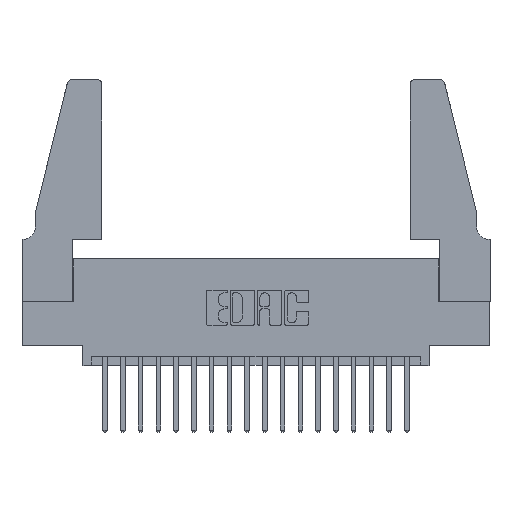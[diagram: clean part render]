
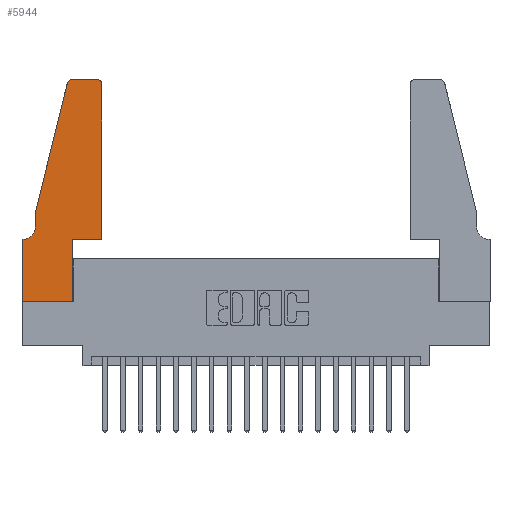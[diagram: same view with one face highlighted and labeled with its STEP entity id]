
A CAD part, top view. The second image highlights one B-rep face of the part: STEP entity #5944.
In plain terms, the highlighted planar face has unit normal (0, 0, 1).
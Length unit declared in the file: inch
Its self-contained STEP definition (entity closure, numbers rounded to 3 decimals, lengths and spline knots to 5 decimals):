
#73 = CARTESIAN_POINT ( 'NONE',  ( 0.2605, 1.25, 0.37 ) ) ;
#491 = DIRECTION ( 'NONE',  ( 0., -1., 0. ) ) ;
#494 = LINE ( 'NONE', #3591, #12289 ) ;
#753 = CARTESIAN_POINT ( 'NONE',  ( 0.2865, 0.35, 0.37 ) ) ;
#868 = CARTESIAN_POINT ( 'NONE',  ( 0.284, 1.22, 0.37 ) ) ;
#1117 = DIRECTION ( 'NONE',  ( -1., 0., 0. ) ) ;
#1159 = LINE ( 'NONE', #73, #8864 ) ;
#1580 = LINE ( 'NONE', #13448, #9281 ) ;
#1698 = DIRECTION ( 'NONE',  ( 0., 1., 0. ) ) ;
#1801 = ORIENTED_EDGE ( 'NONE', *, *, #15707, .T. ) ;
#1884 = CARTESIAN_POINT ( 'NONE',  ( 0.2865, 0., 0.37 ) ) ;
#2112 = ORIENTED_EDGE ( 'NONE', *, *, #2718, .T. ) ;
#2433 = DIRECTION ( 'NONE',  ( 1., 0., 0. ) ) ;
#2710 = DIRECTION ( 'NONE',  ( 0., 1., 0. ) ) ;
#2718 = EDGE_CURVE ( 'NONE', #13651, #10757, #12244, .T. ) ;
#3139 = DIRECTION ( 'NONE',  ( -1., 0., 0. ) ) ;
#3528 = ORIENTED_EDGE ( 'NONE', *, *, #18840, .T. ) ;
#3591 = CARTESIAN_POINT ( 'NONE',  ( 0., 0., 0.37 ) ) ;
#3637 = AXIS2_PLACEMENT_3D ( 'NONE', #19285, #10341, #1117 ) ;
#3677 = CARTESIAN_POINT ( 'NONE',  ( 0.4205, 1.22, 0.37 ) ) ;
#3993 = CARTESIAN_POINT ( 'NONE',  ( 0.0755, 0.5, 0.37 ) ) ;
#4650 = ORIENTED_EDGE ( 'NONE', *, *, #13378, .T. ) ;
#4763 = CARTESIAN_POINT ( 'NONE',  ( 0.4505, 0.35, 0.37 ) ) ;
#4810 = EDGE_CURVE ( 'NONE', #14926, #13351, #1580, .T. ) ;
#5226 = DIRECTION ( 'NONE',  ( 1., 0., 0. ) ) ;
#5566 = DIRECTION ( 'NONE',  ( 0., -1., 0. ) ) ;
#5788 = DIRECTION ( 'NONE',  ( -0.239, -0.971, 0. ) ) ;
#5944 = ADVANCED_FACE ( 'NONE', ( #18175 ), #12454, .T. ) ;
#6122 = VECTOR ( 'NONE', #19606, 39.37008 ) ;
#6267 = AXIS2_PLACEMENT_3D ( 'NONE', #3677, #14351, #5226 ) ;
#6272 = CARTESIAN_POINT ( 'NONE',  ( 0.2865, 0.35, 0.37 ) ) ;
#6332 = DIRECTION ( 'NONE',  ( 1., 0., 0. ) ) ;
#6452 = CARTESIAN_POINT ( 'NONE',  ( 0., 0.35, 0.37 ) ) ;
#6780 = ORIENTED_EDGE ( 'NONE', *, *, #13356, .T. ) ;
#7181 = CARTESIAN_POINT ( 'NONE',  ( 0.4205, 1.25, 0.37 ) ) ;
#7207 = AXIS2_PLACEMENT_3D ( 'NONE', #13944, #15433, #6332 ) ;
#7335 = EDGE_CURVE ( 'NONE', #10085, #14926, #16744, .T. ) ;
#7605 = LINE ( 'NONE', #14009, #10738 ) ;
#8207 = VERTEX_POINT ( 'NONE', #18926 ) ;
#8531 = CARTESIAN_POINT ( 'NONE',  ( 0.0755, 0.42, 0.37 ) ) ;
#8585 = VERTEX_POINT ( 'NONE', #10897 ) ;
#8630 = VECTOR ( 'NONE', #5566, 39.37008 ) ;
#8864 = VECTOR ( 'NONE', #3139, 39.37008 ) ;
#8877 = CARTESIAN_POINT ( 'NONE',  ( 0.4505, 0.35, 0.37 ) ) ;
#9092 = ORIENTED_EDGE ( 'NONE', *, *, #14927, .T. ) ;
#9281 = VECTOR ( 'NONE', #2710, 39.37008 ) ;
#9376 = DIRECTION ( 'NONE',  ( 1., 0., 0. ) ) ;
#9969 = EDGE_CURVE ( 'NONE', #12098, #10286, #494, .T. ) ;
#10085 = VERTEX_POINT ( 'NONE', #753 ) ;
#10138 = ORIENTED_EDGE ( 'NONE', *, *, #7335, .T. ) ;
#10286 = VERTEX_POINT ( 'NONE', #19382 ) ;
#10341 = DIRECTION ( 'NONE',  ( 0., 0., -1. ) ) ;
#10649 = VECTOR ( 'NONE', #9376, 39.37008 ) ;
#10738 = VECTOR ( 'NONE', #15509, 39.37008 ) ;
#10757 = VERTEX_POINT ( 'NONE', #8531 ) ;
#10801 = ORIENTED_EDGE ( 'NONE', *, *, #17772, .T. ) ;
#10897 = CARTESIAN_POINT ( 'NONE',  ( 0.25487, 1.22718, 0.37 ) ) ;
#11215 = VECTOR ( 'NONE', #1698, 39.37008 ) ;
#11423 = ORIENTED_EDGE ( 'NONE', *, *, #4810, .T. ) ;
#11634 = DIRECTION ( 'NONE',  ( 0., 0., 1. ) ) ;
#11692 = LINE ( 'NONE', #6272, #11215 ) ;
#11838 = ORIENTED_EDGE ( 'NONE', *, *, #9969, .T. ) ;
#12098 = VERTEX_POINT ( 'NONE', #6452 ) ;
#12122 = CIRCLE ( 'NONE', #15082, 0.03 ) ;
#12153 = ORIENTED_EDGE ( 'NONE', *, *, #15891, .T. ) ;
#12244 = LINE ( 'NONE', #16173, #8630 ) ;
#12252 = CARTESIAN_POINT ( 'NONE',  ( 0.0055, 0.35, 0.37 ) ) ;
#12289 = VECTOR ( 'NONE', #491, 39.37008 ) ;
#12350 = CARTESIAN_POINT ( 'NONE',  ( 0.4505, 1.22, 0.37 ) ) ;
#12396 = EDGE_CURVE ( 'NONE', #10757, #13307, #17568, .T. ) ;
#12454 = PLANE ( 'NONE',  #7207 ) ;
#12497 = ORIENTED_EDGE ( 'NONE', *, *, #12396, .T. ) ;
#12512 = VECTOR ( 'NONE', #5788, 39.37008 ) ;
#13307 = VERTEX_POINT ( 'NONE', #12252 ) ;
#13351 = VERTEX_POINT ( 'NONE', #12350 ) ;
#13356 = EDGE_CURVE ( 'NONE', #17335, #10085, #11692, .T. ) ;
#13378 = EDGE_CURVE ( 'NONE', #10286, #17335, #7605, .T. ) ;
#13448 = CARTESIAN_POINT ( 'NONE',  ( 0.4505, 0.35, 0.37 ) ) ;
#13651 = VERTEX_POINT ( 'NONE', #3993 ) ;
#13944 = CARTESIAN_POINT ( 'NONE',  ( 0., 0.35, 0.37 ) ) ;
#14009 = CARTESIAN_POINT ( 'NONE',  ( 0., 0., 0.37 ) ) ;
#14351 = DIRECTION ( 'NONE',  ( 0., 0., 1. ) ) ;
#14926 = VERTEX_POINT ( 'NONE', #8877 ) ;
#14927 = EDGE_CURVE ( 'NONE', #8585, #13651, #16444, .T. ) ;
#15082 = AXIS2_PLACEMENT_3D ( 'NONE', #868, #11634, #2433 ) ;
#15433 = DIRECTION ( 'NONE',  ( 0., 0., 1. ) ) ;
#15509 = DIRECTION ( 'NONE',  ( 1., 0., 0. ) ) ;
#15707 = EDGE_CURVE ( 'NONE', #17616, #8207, #1159, .T. ) ;
#15891 = EDGE_CURVE ( 'NONE', #13351, #17616, #17114, .T. ) ;
#16173 = CARTESIAN_POINT ( 'NONE',  ( 0.0755, 0.5, 0.37 ) ) ;
#16392 = CARTESIAN_POINT ( 'NONE',  ( 0.0755, 0.5, 0.37 ) ) ;
#16444 = LINE ( 'NONE', #16392, #12512 ) ;
#16744 = LINE ( 'NONE', #4763, #10649 ) ;
#17114 = CIRCLE ( 'NONE', #6267, 0.03 ) ;
#17335 = VERTEX_POINT ( 'NONE', #1884 ) ;
#17568 = CIRCLE ( 'NONE', #3637, 0.07 ) ;
#17616 = VERTEX_POINT ( 'NONE', #7181 ) ;
#17772 = EDGE_CURVE ( 'NONE', #13307, #12098, #18164, .T. ) ;
#17824 = EDGE_LOOP ( 'NONE', ( #1801, #3528, #9092, #2112, #12497, #10801, #11838, #4650, #6780, #10138, #11423, #12153 ) ) ;
#18118 = CARTESIAN_POINT ( 'NONE',  ( 0.0755, 0.35, 0.37 ) ) ;
#18164 = LINE ( 'NONE', #18118, #6122 ) ;
#18175 = FACE_OUTER_BOUND ( 'NONE', #17824, .T. ) ;
#18840 = EDGE_CURVE ( 'NONE', #8207, #8585, #12122, .T. ) ;
#18926 = CARTESIAN_POINT ( 'NONE',  ( 0.284, 1.25, 0.37 ) ) ;
#19285 = CARTESIAN_POINT ( 'NONE',  ( 0.0055, 0.42, 0.37 ) ) ;
#19382 = CARTESIAN_POINT ( 'NONE',  ( 0., 0., 0.37 ) ) ;
#19606 = DIRECTION ( 'NONE',  ( -1., 0., 0. ) ) ;
